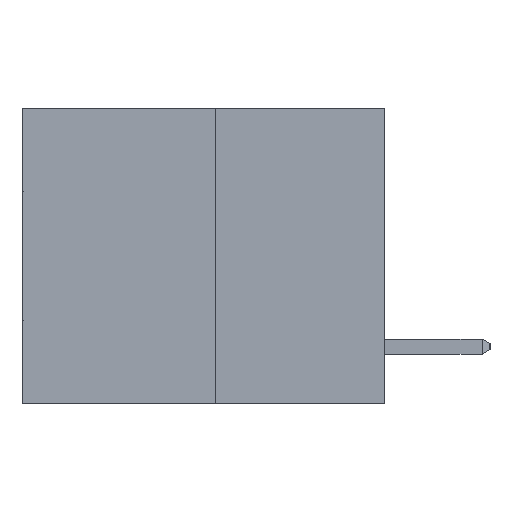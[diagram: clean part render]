
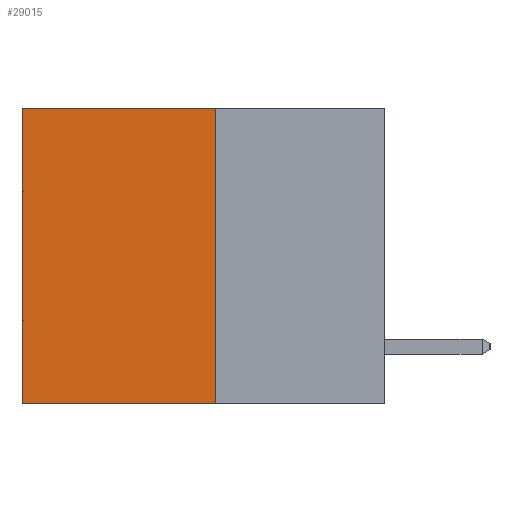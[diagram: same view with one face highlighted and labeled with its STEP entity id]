
A CAD part, left-side view. The second image highlights one B-rep face of the part: STEP entity #29015.
In plain terms, the highlighted planar face has unit normal (-1, 0, 0).
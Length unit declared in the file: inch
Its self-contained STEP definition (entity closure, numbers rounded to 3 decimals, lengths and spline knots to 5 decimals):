
#978 = DIRECTION ( 'NONE',  ( 0., 1., 0. ) ) ;
#1465 = CARTESIAN_POINT ( 'NONE',  ( 0.3165, 0.6, -0.49 ) ) ;
#1470 = FACE_OUTER_BOUND ( 'NONE', #22743, .T. ) ;
#4143 = CARTESIAN_POINT ( 'NONE',  ( 0.3165, 0.28, -0.49 ) ) ;
#5193 = DIRECTION ( 'NONE',  ( 1., 0., 0. ) ) ;
#5343 = CARTESIAN_POINT ( 'NONE',  ( 0.3165, 0.6, -0.49 ) ) ;
#5507 = EDGE_CURVE ( 'NONE', #9369, #17337, #8207, .T. ) ;
#5955 = VECTOR ( 'NONE', #19657, 39.37008 ) ;
#6821 = LINE ( 'NONE', #23746, #18107 ) ;
#7449 = CARTESIAN_POINT ( 'NONE',  ( 0.3165, 0.28, -0.49 ) ) ;
#8207 = LINE ( 'NONE', #28928, #24030 ) ;
#9369 = VERTEX_POINT ( 'NONE', #25099 ) ;
#13879 = AXIS2_PLACEMENT_3D ( 'NONE', #7449, #5193, #27585 ) ;
#15810 = VECTOR ( 'NONE', #16190, 39.37008 ) ;
#16190 = DIRECTION ( 'NONE',  ( 0., 0., -1. ) ) ;
#16687 = CARTESIAN_POINT ( 'NONE',  ( 0.3165, 0.6, 0. ) ) ;
#16722 = ORIENTED_EDGE ( 'NONE', *, *, #21053, .T. ) ;
#17337 = VERTEX_POINT ( 'NONE', #16687 ) ;
#18107 = VECTOR ( 'NONE', #978, 39.37008 ) ;
#18555 = LINE ( 'NONE', #19566, #5955 ) ;
#18939 = ORIENTED_EDGE ( 'NONE', *, *, #5507, .T. ) ;
#19566 = CARTESIAN_POINT ( 'NONE',  ( 0.3165, 0.28, -0.49 ) ) ;
#19657 = DIRECTION ( 'NONE',  ( 0., 0., -1. ) ) ;
#21053 = EDGE_CURVE ( 'NONE', #17337, #22487, #21824, .T. ) ;
#21824 = LINE ( 'NONE', #5343, #15810 ) ;
#21888 = ORIENTED_EDGE ( 'NONE', *, *, #22986, .F. ) ;
#22487 = VERTEX_POINT ( 'NONE', #1465 ) ;
#22605 = DIRECTION ( 'NONE',  ( 0., 1., 0. ) ) ;
#22743 = EDGE_LOOP ( 'NONE', ( #16722, #27969, #21888, #18939 ) ) ;
#22986 = EDGE_CURVE ( 'NONE', #9369, #24550, #18555, .T. ) ;
#23048 = PLANE ( 'NONE',  #13879 ) ;
#23746 = CARTESIAN_POINT ( 'NONE',  ( 0.3165, 0.28, -0.49 ) ) ;
#24030 = VECTOR ( 'NONE', #22605, 39.37008 ) ;
#24550 = VERTEX_POINT ( 'NONE', #4143 ) ;
#24846 = EDGE_CURVE ( 'NONE', #24550, #22487, #6821, .T. ) ;
#25099 = CARTESIAN_POINT ( 'NONE',  ( 0.3165, 0.28, 0. ) ) ;
#27585 = DIRECTION ( 'NONE',  ( 0., 0., -1. ) ) ;
#27969 = ORIENTED_EDGE ( 'NONE', *, *, #24846, .F. ) ;
#28928 = CARTESIAN_POINT ( 'NONE',  ( 0.3165, 0.28, 0. ) ) ;
#29015 = ADVANCED_FACE ( 'NONE', ( #1470 ), #23048, .F. ) ;
